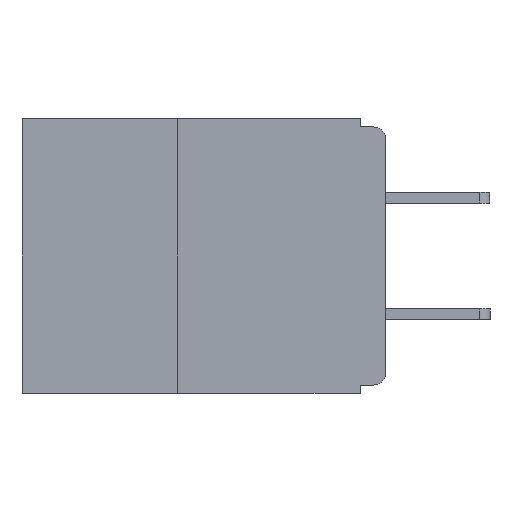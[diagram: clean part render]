
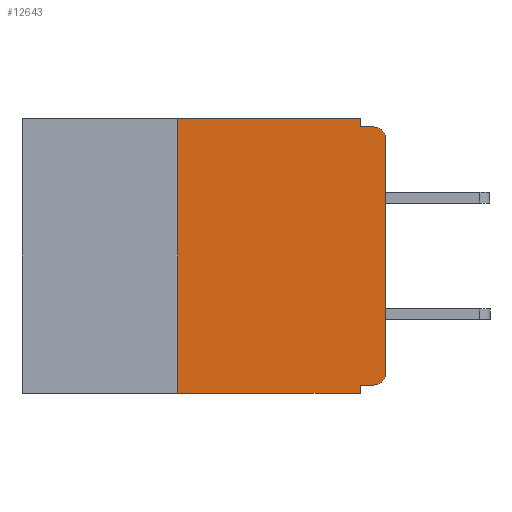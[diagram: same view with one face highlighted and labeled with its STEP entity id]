
A CAD part, left-side view. The second image highlights one B-rep face of the part: STEP entity #12643.
In plain terms, the highlighted planar face has unit normal (-1, 0, 0).
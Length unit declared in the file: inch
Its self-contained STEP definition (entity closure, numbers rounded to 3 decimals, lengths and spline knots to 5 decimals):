
#136 = EDGE_CURVE ( 'NONE', #4931, #5021, #841, .T. ) ;
#249 = DIRECTION ( 'NONE',  ( -1., 0., 0. ) ) ;
#288 = CARTESIAN_POINT ( 'NONE',  ( 0., 0.015, -0.01 ) ) ;
#841 = CIRCLE ( 'NONE', #11698, 0.015 ) ;
#844 = LINE ( 'NONE', #8690, #11789 ) ;
#1126 = ORIENTED_EDGE ( 'NONE', *, *, #15752, .F. ) ;
#1347 = ORIENTED_EDGE ( 'NONE', *, *, #16688, .F. ) ;
#1353 = CARTESIAN_POINT ( 'NONE',  ( 0., 0.25, 0. ) ) ;
#1436 = VERTEX_POINT ( 'NONE', #16929 ) ;
#1525 = LINE ( 'NONE', #15126, #8324 ) ;
#1535 = ORIENTED_EDGE ( 'NONE', *, *, #9337, .T. ) ;
#1927 = VECTOR ( 'NONE', #17172, 39.37008 ) ;
#1955 = ORIENTED_EDGE ( 'NONE', *, *, #2746, .T. ) ;
#1993 = LINE ( 'NONE', #4909, #8816 ) ;
#2374 = LINE ( 'NONE', #7715, #12860 ) ;
#2418 = DIRECTION ( 'NONE',  ( 0., 0., 1. ) ) ;
#2746 = EDGE_CURVE ( 'NONE', #2955, #4931, #1525, .T. ) ;
#2955 = VERTEX_POINT ( 'NONE', #6645 ) ;
#3708 = AXIS2_PLACEMENT_3D ( 'NONE', #15544, #15481, #15450 ) ;
#4528 = AXIS2_PLACEMENT_3D ( 'NONE', #8109, #8076, #8059 ) ;
#4909 = CARTESIAN_POINT ( 'NONE',  ( 0., 0.437, -0.33 ) ) ;
#4928 = DIRECTION ( 'NONE',  ( 0., -1., 0. ) ) ;
#4931 = VERTEX_POINT ( 'NONE', #5595 ) ;
#5021 = VERTEX_POINT ( 'NONE', #288 ) ;
#5165 = VERTEX_POINT ( 'NONE', #15120 ) ;
#5233 = VERTEX_POINT ( 'NONE', #13554 ) ;
#5595 = CARTESIAN_POINT ( 'NONE',  ( 0., 0., -0.025 ) ) ;
#5596 = LINE ( 'NONE', #11646, #9238 ) ;
#5974 = LINE ( 'NONE', #10551, #1927 ) ;
#6132 = VECTOR ( 'NONE', #9372, 39.37008 ) ;
#6579 = EDGE_CURVE ( 'NONE', #5165, #7801, #11236, .T. ) ;
#6645 = CARTESIAN_POINT ( 'NONE',  ( 0., 0., -0.305 ) ) ;
#6764 = CARTESIAN_POINT ( 'NONE',  ( 0., 0.015, -0.025 ) ) ;
#7131 = ORIENTED_EDGE ( 'NONE', *, *, #13345, .F. ) ;
#7306 = ORIENTED_EDGE ( 'NONE', *, *, #136, .T. ) ;
#7308 = CARTESIAN_POINT ( 'NONE',  ( 0., 0.031, -0.33 ) ) ;
#7542 = ORIENTED_EDGE ( 'NONE', *, *, #10727, .F. ) ;
#7552 = DIRECTION ( 'NONE',  ( 0., 1., 0. ) ) ;
#7573 = VECTOR ( 'NONE', #11473, 39.37008 ) ;
#7715 = CARTESIAN_POINT ( 'NONE',  ( 0., 0., -0.32 ) ) ;
#7801 = VERTEX_POINT ( 'NONE', #1353 ) ;
#8059 = DIRECTION ( 'NONE',  ( 0., 0., -1. ) ) ;
#8076 = DIRECTION ( 'NONE',  ( -1., 0., 0. ) ) ;
#8082 = CARTESIAN_POINT ( 'NONE',  ( 0., 0.015, -0.32 ) ) ;
#8109 = CARTESIAN_POINT ( 'NONE',  ( 0., 0.015, -0.305 ) ) ;
#8324 = VECTOR ( 'NONE', #2418, 39.37008 ) ;
#8466 = CIRCLE ( 'NONE', #4528, 0.015 ) ;
#8690 = CARTESIAN_POINT ( 'NONE',  ( 0., 0.437, 0. ) ) ;
#8807 = VERTEX_POINT ( 'NONE', #17322 ) ;
#8816 = VECTOR ( 'NONE', #4928, 39.37008 ) ;
#9238 = VECTOR ( 'NONE', #11643, 39.37008 ) ;
#9337 = EDGE_CURVE ( 'NONE', #5165, #16113, #1993, .T. ) ;
#9372 = DIRECTION ( 'NONE',  ( 0., 0., -1. ) ) ;
#9878 = CARTESIAN_POINT ( 'NONE',  ( 0., 0.031, -0.33 ) ) ;
#10262 = EDGE_CURVE ( 'NONE', #8807, #5233, #5596, .T. ) ;
#10551 = CARTESIAN_POINT ( 'NONE',  ( 0., 0., -0.01 ) ) ;
#10727 = EDGE_CURVE ( 'NONE', #16986, #1436, #2374, .T. ) ;
#11236 = LINE ( 'NONE', #11546, #7573 ) ;
#11338 = FACE_OUTER_BOUND ( 'NONE', #15182, .T. ) ;
#11473 = DIRECTION ( 'NONE',  ( 0., 0., 1. ) ) ;
#11546 = CARTESIAN_POINT ( 'NONE',  ( 0., 0.25, -0.33 ) ) ;
#11643 = DIRECTION ( 'NONE',  ( 0., 0., -1. ) ) ;
#11646 = CARTESIAN_POINT ( 'NONE',  ( 0., 0.031, 0. ) ) ;
#11698 = AXIS2_PLACEMENT_3D ( 'NONE', #6764, #249, #15984 ) ;
#11789 = VECTOR ( 'NONE', #16756, 39.37008 ) ;
#12643 = ADVANCED_FACE ( 'NONE', ( #11338 ), #15734, .F. ) ;
#12860 = VECTOR ( 'NONE', #7552, 39.37008 ) ;
#13314 = ORIENTED_EDGE ( 'NONE', *, *, #10262, .F. ) ;
#13345 = EDGE_CURVE ( 'NONE', #1436, #16113, #16836, .T. ) ;
#13356 = ORIENTED_EDGE ( 'NONE', *, *, #6579, .F. ) ;
#13461 = EDGE_CURVE ( 'NONE', #16986, #2955, #8466, .T. ) ;
#13554 = CARTESIAN_POINT ( 'NONE',  ( 0., 0.031, -0.01 ) ) ;
#14664 = ORIENTED_EDGE ( 'NONE', *, *, #13461, .T. ) ;
#15120 = CARTESIAN_POINT ( 'NONE',  ( 0., 0.25, -0.33 ) ) ;
#15126 = CARTESIAN_POINT ( 'NONE',  ( 0., 0., 0. ) ) ;
#15182 = EDGE_LOOP ( 'NONE', ( #1955, #7306, #1126, #13314, #1347, #13356, #1535, #7131, #7542, #14664 ) ) ;
#15450 = DIRECTION ( 'NONE',  ( 0., 0., -1. ) ) ;
#15481 = DIRECTION ( 'NONE',  ( 1., 0., 0. ) ) ;
#15544 = CARTESIAN_POINT ( 'NONE',  ( 0., 0.437, 0. ) ) ;
#15734 = PLANE ( 'NONE',  #3708 ) ;
#15752 = EDGE_CURVE ( 'NONE', #5233, #5021, #5974, .T. ) ;
#15984 = DIRECTION ( 'NONE',  ( 0., 0., -1. ) ) ;
#16113 = VERTEX_POINT ( 'NONE', #7308 ) ;
#16688 = EDGE_CURVE ( 'NONE', #7801, #8807, #844, .T. ) ;
#16756 = DIRECTION ( 'NONE',  ( 0., -1., 0. ) ) ;
#16836 = LINE ( 'NONE', #9878, #6132 ) ;
#16929 = CARTESIAN_POINT ( 'NONE',  ( 0., 0.031, -0.32 ) ) ;
#16986 = VERTEX_POINT ( 'NONE', #8082 ) ;
#17172 = DIRECTION ( 'NONE',  ( 0., -1., 0. ) ) ;
#17322 = CARTESIAN_POINT ( 'NONE',  ( 0., 0.031, 0. ) ) ;
